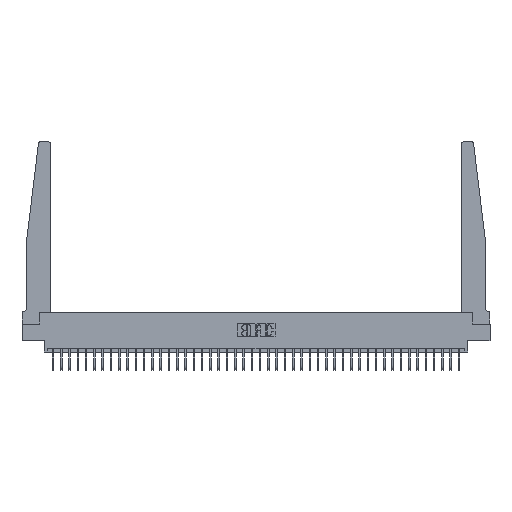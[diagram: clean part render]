
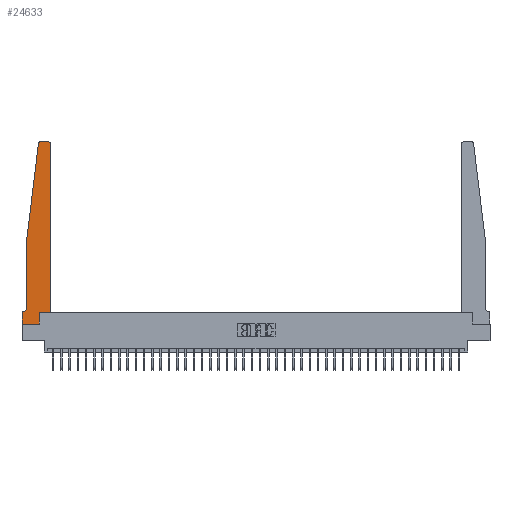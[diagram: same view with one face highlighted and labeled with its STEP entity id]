
A CAD part, top view. The second image highlights one B-rep face of the part: STEP entity #24633.
In plain terms, the highlighted planar face has unit normal (0, 0, 1).
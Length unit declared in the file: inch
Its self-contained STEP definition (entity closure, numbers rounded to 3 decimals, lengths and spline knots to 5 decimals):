
#879 = EDGE_CURVE ( 'NONE', #12071, #13091, #9720, .T. ) ;
#934 = VERTEX_POINT ( 'NONE', #32855 ) ;
#1497 = EDGE_LOOP ( 'NONE', ( #5215, #4470, #18113, #29373, #34439, #21495, #36312, #8696, #22053, #14944, #35894, #15408 ) ) ;
#2340 = PLANE ( 'NONE',  #31621 ) ;
#2486 = DIRECTION ( 'NONE',  ( -0.122, -0.992, 0. ) ) ;
#3435 = VECTOR ( 'NONE', #28600, 39.37008 ) ;
#3593 = VERTEX_POINT ( 'NONE', #16769 ) ;
#3743 = DIRECTION ( 'NONE',  ( 0., 0., 1. ) ) ;
#4470 = ORIENTED_EDGE ( 'NONE', *, *, #17659, .T. ) ;
#4561 = VERTEX_POINT ( 'NONE', #37679 ) ;
#4693 = LINE ( 'NONE', #22894, #3435 ) ;
#4790 = EDGE_CURVE ( 'NONE', #5887, #31073, #15532, .T. ) ;
#4959 = CARTESIAN_POINT ( 'NONE',  ( 0.425, 0.18, 0.37 ) ) ;
#5215 = ORIENTED_EDGE ( 'NONE', *, *, #7127, .T. ) ;
#5305 = LINE ( 'NONE', #17264, #27276 ) ;
#5667 = CIRCLE ( 'NONE', #21922, 0.03 ) ;
#5887 = VERTEX_POINT ( 'NONE', #14915 ) ;
#6640 = CARTESIAN_POINT ( 'NONE',  ( 0.27653, 2.75, 0.37 ) ) ;
#6696 = VECTOR ( 'NONE', #18365, 39.37008 ) ;
#7127 = EDGE_CURVE ( 'NONE', #31073, #29875, #26710, .T. ) ;
#7637 = DIRECTION ( 'NONE',  ( 1., 0., 0. ) ) ;
#7874 = DIRECTION ( 'NONE',  ( 0., -1., 0. ) ) ;
#8481 = VECTOR ( 'NONE', #11810, 39.37008 ) ;
#8696 = ORIENTED_EDGE ( 'NONE', *, *, #21515, .T. ) ;
#9028 = CARTESIAN_POINT ( 'NONE',  ( 0.065, 0.2375, 0.37 ) ) ;
#9674 = LINE ( 'NONE', #27715, #38333 ) ;
#9720 = LINE ( 'NONE', #24031, #6696 ) ;
#9727 = CARTESIAN_POINT ( 'NONE',  ( 0.24675, 2.72367, 0.37 ) ) ;
#10277 = CARTESIAN_POINT ( 'NONE',  ( 0.2605, 0.18, 0.37 ) ) ;
#10907 = EDGE_CURVE ( 'NONE', #28505, #14183, #29311, .T. ) ;
#11201 = DIRECTION ( 'NONE',  ( -1., 0., 0. ) ) ;
#11300 = VERTEX_POINT ( 'NONE', #9028 ) ;
#11656 = CIRCLE ( 'NONE', #25465, 0.05 ) ;
#11810 = DIRECTION ( 'NONE',  ( -1., 0., 0. ) ) ;
#12071 = VERTEX_POINT ( 'NONE', #26776 ) ;
#13091 = VERTEX_POINT ( 'NONE', #35308 ) ;
#14155 = LINE ( 'NONE', #4959, #23228 ) ;
#14183 = VERTEX_POINT ( 'NONE', #18574 ) ;
#14264 = DIRECTION ( 'NONE',  ( 0., 0., 1. ) ) ;
#14778 = CARTESIAN_POINT ( 'NONE',  ( 0.065, 1.25, 0.37 ) ) ;
#14915 = CARTESIAN_POINT ( 'NONE',  ( 0.425, 2.72, 0.37 ) ) ;
#14944 = ORIENTED_EDGE ( 'NONE', *, *, #38115, .T. ) ;
#15408 = ORIENTED_EDGE ( 'NONE', *, *, #4790, .T. ) ;
#15532 = CIRCLE ( 'NONE', #24290, 0.03 ) ;
#15671 = DIRECTION ( 'NONE',  ( 1., 0., 0. ) ) ;
#16028 = VECTOR ( 'NONE', #7874, 39.37008 ) ;
#16769 = CARTESIAN_POINT ( 'NONE',  ( 0.425, 0.18, 0.37 ) ) ;
#16899 = DIRECTION ( 'NONE',  ( 1., 0., 0. ) ) ;
#17264 = CARTESIAN_POINT ( 'NONE',  ( 0.065, 1.25, 0.37 ) ) ;
#17659 = EDGE_CURVE ( 'NONE', #29875, #28505, #5667, .T. ) ;
#18113 = ORIENTED_EDGE ( 'NONE', *, *, #10907, .T. ) ;
#18365 = DIRECTION ( 'NONE',  ( -1., 0., 0. ) ) ;
#18574 = CARTESIAN_POINT ( 'NONE',  ( 0.065, 1.25, 0.37 ) ) ;
#19644 = CARTESIAN_POINT ( 'NONE',  ( 0., 0., 0.37 ) ) ;
#19716 = LINE ( 'NONE', #23234, #20986 ) ;
#20986 = VECTOR ( 'NONE', #38139, 39.37008 ) ;
#21495 = ORIENTED_EDGE ( 'NONE', *, *, #879, .T. ) ;
#21515 = EDGE_CURVE ( 'NONE', #4561, #934, #9674, .T. ) ;
#21922 = AXIS2_PLACEMENT_3D ( 'NONE', #33005, #35761, #27526 ) ;
#22053 = ORIENTED_EDGE ( 'NONE', *, *, #25043, .T. ) ;
#22894 = CARTESIAN_POINT ( 'NONE',  ( 0.425, 0.18, 0.37 ) ) ;
#23228 = VECTOR ( 'NONE', #16899, 39.37008 ) ;
#23234 = CARTESIAN_POINT ( 'NONE',  ( 0.2605, 0.18, 0.37 ) ) ;
#24031 = CARTESIAN_POINT ( 'NONE',  ( 0.065, 0.1875, 0.37 ) ) ;
#24290 = AXIS2_PLACEMENT_3D ( 'NONE', #30596, #3743, #15671 ) ;
#24633 = ADVANCED_FACE ( 'NONE', ( #25861 ), #2340, .T. ) ;
#24634 = EDGE_CURVE ( 'NONE', #3593, #5887, #4693, .T. ) ;
#25043 = EDGE_CURVE ( 'NONE', #934, #29237, #19716, .T. ) ;
#25465 = AXIS2_PLACEMENT_3D ( 'NONE', #38064, #35503, #11201 ) ;
#25481 = EDGE_CURVE ( 'NONE', #14183, #11300, #5305, .T. ) ;
#25861 = FACE_OUTER_BOUND ( 'NONE', #1497, .T. ) ;
#26710 = LINE ( 'NONE', #33370, #8481 ) ;
#26776 = CARTESIAN_POINT ( 'NONE',  ( 0.015, 0.1875, 0.37 ) ) ;
#27276 = VECTOR ( 'NONE', #31471, 39.37008 ) ;
#27526 = DIRECTION ( 'NONE',  ( 1., 0., 0. ) ) ;
#27715 = CARTESIAN_POINT ( 'NONE',  ( 0., 0., 0.37 ) ) ;
#28102 = DIRECTION ( 'NONE',  ( 1., 0., 0. ) ) ;
#28505 = VERTEX_POINT ( 'NONE', #9727 ) ;
#28600 = DIRECTION ( 'NONE',  ( 0., 1., 0. ) ) ;
#28880 = VECTOR ( 'NONE', #2486, 39.37008 ) ;
#29237 = VERTEX_POINT ( 'NONE', #10277 ) ;
#29311 = LINE ( 'NONE', #14778, #28880 ) ;
#29373 = ORIENTED_EDGE ( 'NONE', *, *, #25481, .T. ) ;
#29875 = VERTEX_POINT ( 'NONE', #6640 ) ;
#30409 = CARTESIAN_POINT ( 'NONE',  ( 0.395, 2.75, 0.37 ) ) ;
#30596 = CARTESIAN_POINT ( 'NONE',  ( 0.395, 2.72, 0.37 ) ) ;
#30730 = EDGE_CURVE ( 'NONE', #13091, #4561, #37683, .T. ) ;
#30833 = EDGE_CURVE ( 'NONE', #11300, #12071, #11656, .T. ) ;
#31073 = VERTEX_POINT ( 'NONE', #30409 ) ;
#31471 = DIRECTION ( 'NONE',  ( 0., -1., 0. ) ) ;
#31621 = AXIS2_PLACEMENT_3D ( 'NONE', #34489, #14264, #7637 ) ;
#32855 = CARTESIAN_POINT ( 'NONE',  ( 0.2605, 0., 0.37 ) ) ;
#33005 = CARTESIAN_POINT ( 'NONE',  ( 0.27653, 2.72, 0.37 ) ) ;
#33370 = CARTESIAN_POINT ( 'NONE',  ( 0.25, 2.75, 0.37 ) ) ;
#34439 = ORIENTED_EDGE ( 'NONE', *, *, #30833, .T. ) ;
#34489 = CARTESIAN_POINT ( 'NONE',  ( 0., 0.1875, 0.37 ) ) ;
#35308 = CARTESIAN_POINT ( 'NONE',  ( 0., 0.1875, 0.37 ) ) ;
#35503 = DIRECTION ( 'NONE',  ( 0., 0., -1. ) ) ;
#35761 = DIRECTION ( 'NONE',  ( 0., 0., 1. ) ) ;
#35894 = ORIENTED_EDGE ( 'NONE', *, *, #24634, .T. ) ;
#36312 = ORIENTED_EDGE ( 'NONE', *, *, #30730, .T. ) ;
#37679 = CARTESIAN_POINT ( 'NONE',  ( 0., 0., 0.37 ) ) ;
#37683 = LINE ( 'NONE', #19644, #16028 ) ;
#38064 = CARTESIAN_POINT ( 'NONE',  ( 0.015, 0.2375, 0.37 ) ) ;
#38115 = EDGE_CURVE ( 'NONE', #29237, #3593, #14155, .T. ) ;
#38139 = DIRECTION ( 'NONE',  ( 0., 1., 0. ) ) ;
#38333 = VECTOR ( 'NONE', #28102, 39.37008 ) ;
